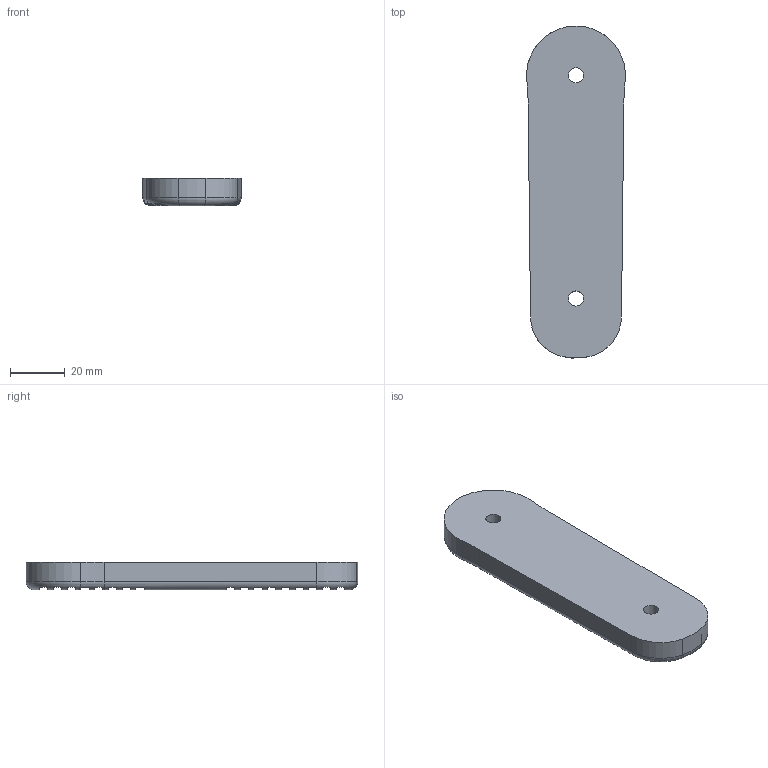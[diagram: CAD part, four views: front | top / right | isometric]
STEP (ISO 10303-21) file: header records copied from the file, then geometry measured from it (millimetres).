
FILE_DESCRIPTION(/* description */ (''),/* implementation_level */ '2;1');
FILE_NAME(/* name */ 'Custom Stock Pad.step',/* time_stamp */ '2022-05-27T20:32:29-05:00',/* author */ (''),/* organization */ (''),/* preprocessor_version */ 'ST-DEVELOPER v19',/* originating_system */ 'Autodesk Translation Framework v11.7.0.108',/* authorisation */ '');
FILE_SCHEMA (('AUTOMOTIVE_DESIGN { 1 0 10303 214 3 1 1 }'));
Length unit declared in the file: millimetre
Products named in the file (1): Custom Stock
Bounding box: 35.9 x 120.92 x 10.04 mm (x, y, z)
Volume: 36132.4 mm3; surface area: 11622.1 mm2
Topology: 1 solids, 1 shells, 198 faces, 571 edges, 377 vertices
Faces by surface type: plane 137, cylinder 55, torus 6
Full cylindrical faces by diameter (mm): 5.5 x2, 10 x2
Entity records: 7363 total; most frequent: CARTESIAN_POINT 2213, ORIENTED_EDGE 1142, DIRECTION 978, EDGE_CURVE 571, VERTEX_POINT 377, LINE 334, VECTOR 334, AXIS2_PLACEMENT_3D 322
